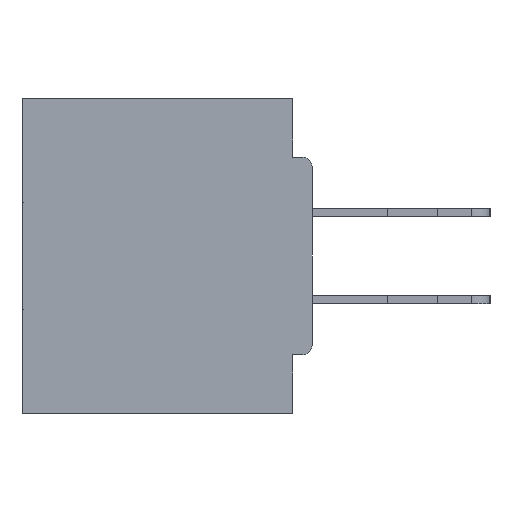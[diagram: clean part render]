
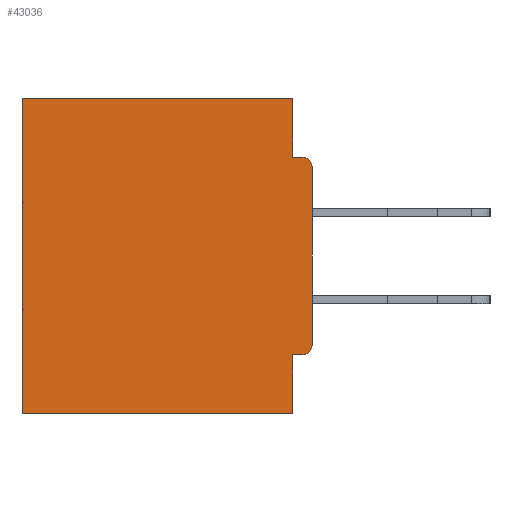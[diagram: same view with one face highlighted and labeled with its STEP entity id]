
A CAD part, left-side view. The second image highlights one B-rep face of the part: STEP entity #43036.
In plain terms, the highlighted planar face has unit normal (-1, 0, 0).
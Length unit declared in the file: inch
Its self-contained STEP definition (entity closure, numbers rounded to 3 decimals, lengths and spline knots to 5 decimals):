
#22 = CIRCLE ( 'NONE', #21047, 0.015 ) ;
#203 = EDGE_CURVE ( 'NONE', #35580, #30565, #42976, .T. ) ;
#656 = VECTOR ( 'NONE', #18358, 39.37008 ) ;
#766 = EDGE_CURVE ( 'NONE', #14672, #2342, #2679, .T. ) ;
#1258 = PLANE ( 'NONE',  #12872 ) ;
#1345 = ORIENTED_EDGE ( 'NONE', *, *, #29648, .F. ) ;
#1393 = DIRECTION ( 'NONE',  ( 0., 0., -1. ) ) ;
#1948 = DIRECTION ( 'NONE',  ( 0., 0., -1. ) ) ;
#2342 = VERTEX_POINT ( 'NONE', #11530 ) ;
#2402 = VERTEX_POINT ( 'NONE', #35603 ) ;
#2679 = LINE ( 'NONE', #13224, #12127 ) ;
#2906 = EDGE_LOOP ( 'NONE', ( #42867, #5344, #1345, #14559, #34618, #6655, #15341, #13840, #14749, #12903 ) ) ;
#3596 = CARTESIAN_POINT ( 'NONE',  ( 0.298, 0., 0. ) ) ;
#4474 = VERTEX_POINT ( 'NONE', #27520 ) ;
#5344 = ORIENTED_EDGE ( 'NONE', *, *, #203, .F. ) ;
#5838 = LINE ( 'NONE', #13842, #39291 ) ;
#6527 = DIRECTION ( 'NONE',  ( 0., 1., 0. ) ) ;
#6655 = ORIENTED_EDGE ( 'NONE', *, *, #40177, .F. ) ;
#8358 = CARTESIAN_POINT ( 'NONE',  ( 0.298, 0.031, 0. ) ) ;
#9773 = CARTESIAN_POINT ( 'NONE',  ( 0.298, 0.031, -0.5 ) ) ;
#10170 = VECTOR ( 'NONE', #12208, 39.37008 ) ;
#11530 = CARTESIAN_POINT ( 'NONE',  ( 0.298, 0.031, -0.4065 ) ) ;
#12127 = VECTOR ( 'NONE', #6527, 39.37008 ) ;
#12173 = DIRECTION ( 'NONE',  ( 0., 1., 0. ) ) ;
#12208 = DIRECTION ( 'NONE',  ( 0., 0., -1. ) ) ;
#12655 = VECTOR ( 'NONE', #19973, 39.37008 ) ;
#12872 = AXIS2_PLACEMENT_3D ( 'NONE', #14736, #18100, #1393 ) ;
#12903 = ORIENTED_EDGE ( 'NONE', *, *, #22400, .F. ) ;
#13044 = VERTEX_POINT ( 'NONE', #17481 ) ;
#13224 = CARTESIAN_POINT ( 'NONE',  ( 0.298, 0., -0.4065 ) ) ;
#13401 = DIRECTION ( 'NONE',  ( 0., 0., -1. ) ) ;
#13840 = ORIENTED_EDGE ( 'NONE', *, *, #766, .F. ) ;
#13842 = CARTESIAN_POINT ( 'NONE',  ( 0.298, 0.46, 0. ) ) ;
#14050 = VERTEX_POINT ( 'NONE', #38571 ) ;
#14559 = ORIENTED_EDGE ( 'NONE', *, *, #19871, .T. ) ;
#14672 = VERTEX_POINT ( 'NONE', #38936 ) ;
#14736 = CARTESIAN_POINT ( 'NONE',  ( 0.298, 0., 0. ) ) ;
#14749 = ORIENTED_EDGE ( 'NONE', *, *, #33064, .T. ) ;
#15127 = DIRECTION ( 'NONE',  ( 0., 0., -1. ) ) ;
#15341 = ORIENTED_EDGE ( 'NONE', *, *, #29345, .F. ) ;
#15353 = VECTOR ( 'NONE', #12173, 39.37008 ) ;
#15410 = DIRECTION ( 'NONE',  ( -1., 0., 0. ) ) ;
#15883 = LINE ( 'NONE', #26060, #10170 ) ;
#16675 = VERTEX_POINT ( 'NONE', #8358 ) ;
#17481 = CARTESIAN_POINT ( 'NONE',  ( 0.298, 0., -0.1085 ) ) ;
#18100 = DIRECTION ( 'NONE',  ( 1., 0., 0. ) ) ;
#18358 = DIRECTION ( 'NONE',  ( 0., -1., 0. ) ) ;
#19068 = CARTESIAN_POINT ( 'NONE',  ( 0.298, 0.015, -0.3915 ) ) ;
#19871 = EDGE_CURVE ( 'NONE', #16675, #2402, #35204, .T. ) ;
#19973 = DIRECTION ( 'NONE',  ( 0., 1., 0. ) ) ;
#21047 = AXIS2_PLACEMENT_3D ( 'NONE', #19068, #15410, #1948 ) ;
#21963 = CIRCLE ( 'NONE', #25711, 0.015 ) ;
#22150 = CARTESIAN_POINT ( 'NONE',  ( 0.298, 0.031, -0.0935 ) ) ;
#22400 = EDGE_CURVE ( 'NONE', #13044, #33918, #15883, .T. ) ;
#23489 = LINE ( 'NONE', #38933, #32927 ) ;
#25274 = LINE ( 'NONE', #32779, #15353 ) ;
#25711 = AXIS2_PLACEMENT_3D ( 'NONE', #31413, #41902, #42037 ) ;
#26060 = CARTESIAN_POINT ( 'NONE',  ( 0.298, 0., 0. ) ) ;
#27105 = DIRECTION ( 'NONE',  ( 0., 0., -1. ) ) ;
#27520 = CARTESIAN_POINT ( 'NONE',  ( 0.298, 0.46, -0.5 ) ) ;
#29345 = EDGE_CURVE ( 'NONE', #2342, #14050, #39730, .T. ) ;
#29648 = EDGE_CURVE ( 'NONE', #16675, #35580, #23489, .T. ) ;
#30565 = VERTEX_POINT ( 'NONE', #38131 ) ;
#31066 = CARTESIAN_POINT ( 'NONE',  ( 0.298, 0., -0.3915 ) ) ;
#31413 = CARTESIAN_POINT ( 'NONE',  ( 0.298, 0.015, -0.1085 ) ) ;
#32779 = CARTESIAN_POINT ( 'NONE',  ( 0.298, 0., -0.5 ) ) ;
#32927 = VECTOR ( 'NONE', #15127, 39.37008 ) ;
#33064 = EDGE_CURVE ( 'NONE', #14672, #33918, #22, .T. ) ;
#33918 = VERTEX_POINT ( 'NONE', #31066 ) ;
#34618 = ORIENTED_EDGE ( 'NONE', *, *, #40954, .T. ) ;
#34977 = FACE_OUTER_BOUND ( 'NONE', #2906, .T. ) ;
#35030 = CARTESIAN_POINT ( 'NONE',  ( 0.298, 0., -0.0935 ) ) ;
#35204 = LINE ( 'NONE', #3596, #12655 ) ;
#35580 = VERTEX_POINT ( 'NONE', #22150 ) ;
#35603 = CARTESIAN_POINT ( 'NONE',  ( 0.298, 0.46, 0. ) ) ;
#38131 = CARTESIAN_POINT ( 'NONE',  ( 0.298, 0.015, -0.0935 ) ) ;
#38571 = CARTESIAN_POINT ( 'NONE',  ( 0.298, 0.031, -0.5 ) ) ;
#38933 = CARTESIAN_POINT ( 'NONE',  ( 0.298, 0.031, -0.5 ) ) ;
#38936 = CARTESIAN_POINT ( 'NONE',  ( 0.298, 0.015, -0.4065 ) ) ;
#39185 = VECTOR ( 'NONE', #13401, 39.37008 ) ;
#39291 = VECTOR ( 'NONE', #27105, 39.37008 ) ;
#39730 = LINE ( 'NONE', #9773, #39185 ) ;
#40177 = EDGE_CURVE ( 'NONE', #14050, #4474, #25274, .T. ) ;
#40954 = EDGE_CURVE ( 'NONE', #2402, #4474, #5838, .T. ) ;
#41855 = EDGE_CURVE ( 'NONE', #13044, #30565, #21963, .T. ) ;
#41902 = DIRECTION ( 'NONE',  ( -1., 0., 0. ) ) ;
#42037 = DIRECTION ( 'NONE',  ( 0., 0., -1. ) ) ;
#42867 = ORIENTED_EDGE ( 'NONE', *, *, #41855, .T. ) ;
#42976 = LINE ( 'NONE', #35030, #656 ) ;
#43036 = ADVANCED_FACE ( 'NONE', ( #34977 ), #1258, .F. ) ;
